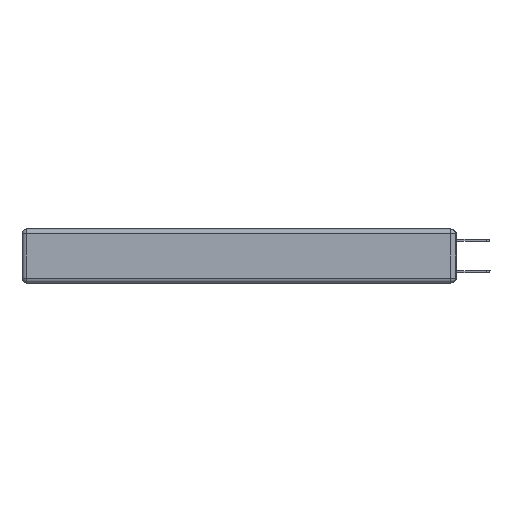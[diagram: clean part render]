
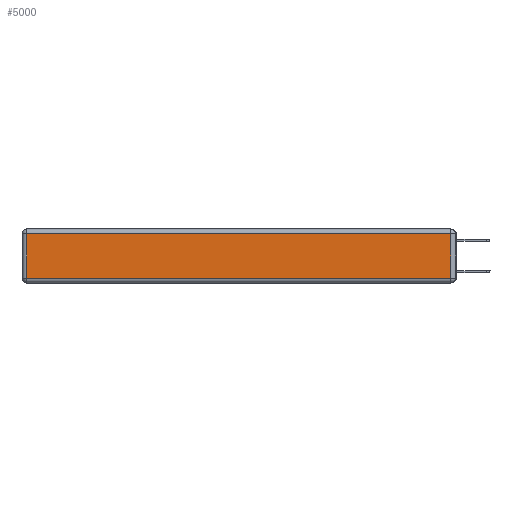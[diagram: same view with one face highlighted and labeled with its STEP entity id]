
A CAD part, left-side view. The second image highlights one B-rep face of the part: STEP entity #5000.
In plain terms, the highlighted planar face has unit normal (-1, 0, 0).
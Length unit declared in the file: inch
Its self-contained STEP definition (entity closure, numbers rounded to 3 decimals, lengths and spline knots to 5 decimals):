
#693 = VECTOR ( 'NONE', #16678, 39.37008 ) ;
#1728 = LINE ( 'NONE', #3103, #20434 ) ;
#2622 = VERTEX_POINT ( 'NONE', #16648 ) ;
#2908 = DIRECTION ( 'NONE',  ( 0., 0., 1. ) ) ;
#3103 = CARTESIAN_POINT ( 'NONE',  ( 0., 0., -0.313 ) ) ;
#3191 = FACE_OUTER_BOUND ( 'NONE', #14438, .T. ) ;
#3751 = CARTESIAN_POINT ( 'NONE',  ( 0., 2.72, -0.343 ) ) ;
#4376 = CARTESIAN_POINT ( 'NONE',  ( 0., 2.75, -0.03 ) ) ;
#5000 = ADVANCED_FACE ( 'NONE', ( #3191 ), #18364, .T. ) ;
#5008 = ORIENTED_EDGE ( 'NONE', *, *, #6786, .T. ) ;
#5205 = ORIENTED_EDGE ( 'NONE', *, *, #7913, .T. ) ;
#5973 = ORIENTED_EDGE ( 'NONE', *, *, #19303, .T. ) ;
#6381 = LINE ( 'NONE', #4376, #14196 ) ;
#6610 = VERTEX_POINT ( 'NONE', #24772 ) ;
#6786 = EDGE_CURVE ( 'NONE', #20411, #6610, #23851, .T. ) ;
#6808 = CARTESIAN_POINT ( 'NONE',  ( 0., 0.03, -0.343 ) ) ;
#7913 = EDGE_CURVE ( 'NONE', #2622, #20411, #1728, .T. ) ;
#10897 = ORIENTED_EDGE ( 'NONE', *, *, #22680, .T. ) ;
#13598 = VERTEX_POINT ( 'NONE', #15578 ) ;
#14196 = VECTOR ( 'NONE', #23651, 39.37008 ) ;
#14438 = EDGE_LOOP ( 'NONE', ( #5205, #5008, #5973, #10897 ) ) ;
#15578 = CARTESIAN_POINT ( 'NONE',  ( 0., 2.72, -0.03 ) ) ;
#16599 = DIRECTION ( 'NONE',  ( -1., 0., 0. ) ) ;
#16648 = CARTESIAN_POINT ( 'NONE',  ( 0., 2.72, -0.313 ) ) ;
#16678 = DIRECTION ( 'NONE',  ( 0., 0., -1. ) ) ;
#16798 = LINE ( 'NONE', #3751, #693 ) ;
#18364 = PLANE ( 'NONE',  #19147 ) ;
#18389 = DIRECTION ( 'NONE',  ( 0., -1., 0. ) ) ;
#19147 = AXIS2_PLACEMENT_3D ( 'NONE', #24127, #16599, #23749 ) ;
#19278 = VECTOR ( 'NONE', #2908, 39.37008 ) ;
#19303 = EDGE_CURVE ( 'NONE', #6610, #13598, #6381, .T. ) ;
#20411 = VERTEX_POINT ( 'NONE', #22184 ) ;
#20434 = VECTOR ( 'NONE', #18389, 39.37008 ) ;
#22184 = CARTESIAN_POINT ( 'NONE',  ( 0., 0.03, -0.313 ) ) ;
#22680 = EDGE_CURVE ( 'NONE', #13598, #2622, #16798, .T. ) ;
#23651 = DIRECTION ( 'NONE',  ( 0., 1., 0. ) ) ;
#23749 = DIRECTION ( 'NONE',  ( 0., 0., 1. ) ) ;
#23851 = LINE ( 'NONE', #6808, #19278 ) ;
#24127 = CARTESIAN_POINT ( 'NONE',  ( 0., 0., -0.343 ) ) ;
#24772 = CARTESIAN_POINT ( 'NONE',  ( 0., 0.03, -0.03 ) ) ;
